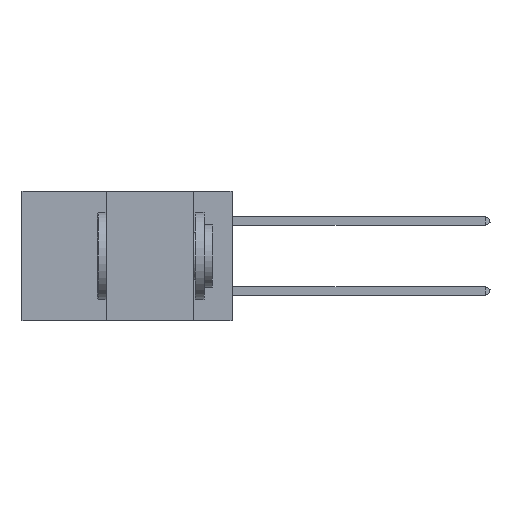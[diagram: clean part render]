
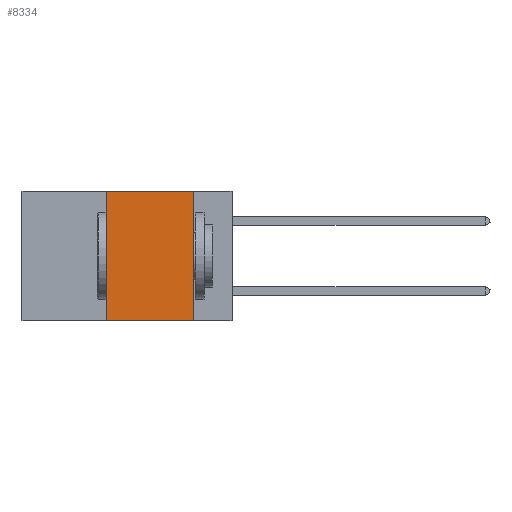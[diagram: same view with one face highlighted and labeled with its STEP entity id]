
A CAD part, left-side view. The second image highlights one B-rep face of the part: STEP entity #8334.
In plain terms, the highlighted planar face has unit normal (-1, 0, 0).
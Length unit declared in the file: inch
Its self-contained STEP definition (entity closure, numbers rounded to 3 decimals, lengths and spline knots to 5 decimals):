
#195 = FACE_OUTER_BOUND ( 'NONE', #5992, .T. ) ;
#325 = VERTEX_POINT ( 'NONE', #12992 ) ;
#503 = DIRECTION ( 'NONE',  ( 0., 0., 1. ) ) ;
#2256 = CARTESIAN_POINT ( 'NONE',  ( 0., 0.36, -0.37 ) ) ;
#2425 = LINE ( 'NONE', #9385, #19684 ) ;
#2683 = CARTESIAN_POINT ( 'NONE',  ( 0., 0.36, 0. ) ) ;
#3695 = EDGE_CURVE ( 'NONE', #325, #13706, #17920, .T. ) ;
#3822 = VERTEX_POINT ( 'NONE', #2256 ) ;
#4269 = EDGE_CURVE ( 'NONE', #20481, #325, #2425, .T. ) ;
#5013 = DIRECTION ( 'NONE',  ( 0., 0., -1. ) ) ;
#5042 = CARTESIAN_POINT ( 'NONE',  ( 0., 0.11, 0. ) ) ;
#5537 = CARTESIAN_POINT ( 'NONE',  ( 0., 0.6, -0.37 ) ) ;
#5992 = EDGE_LOOP ( 'NONE', ( #6625, #15496, #19819, #12196 ) ) ;
#6625 = ORIENTED_EDGE ( 'NONE', *, *, #3695, .F. ) ;
#8334 = ADVANCED_FACE ( 'NONE', ( #195 ), #19979, .F. ) ;
#8519 = DIRECTION ( 'NONE',  ( 0., -1., 0. ) ) ;
#8827 = AXIS2_PLACEMENT_3D ( 'NONE', #16624, #10181, #21620 ) ;
#9231 = VECTOR ( 'NONE', #13923, 39.37008 ) ;
#9385 = CARTESIAN_POINT ( 'NONE',  ( 0., 0.6, 0. ) ) ;
#10110 = CARTESIAN_POINT ( 'NONE',  ( 0., 0.36, 0. ) ) ;
#10181 = DIRECTION ( 'NONE',  ( 1., 0., 0. ) ) ;
#12196 = ORIENTED_EDGE ( 'NONE', *, *, #14826, .T. ) ;
#12992 = CARTESIAN_POINT ( 'NONE',  ( 0., 0.11, 0. ) ) ;
#13103 = VECTOR ( 'NONE', #5013, 39.37008 ) ;
#13273 = VECTOR ( 'NONE', #503, 39.37008 ) ;
#13706 = VERTEX_POINT ( 'NONE', #15265 ) ;
#13923 = DIRECTION ( 'NONE',  ( 0., -1., 0. ) ) ;
#14173 = LINE ( 'NONE', #5537, #9231 ) ;
#14826 = EDGE_CURVE ( 'NONE', #3822, #13706, #14173, .T. ) ;
#15265 = CARTESIAN_POINT ( 'NONE',  ( 0., 0.11, -0.37 ) ) ;
#15496 = ORIENTED_EDGE ( 'NONE', *, *, #4269, .F. ) ;
#16624 = CARTESIAN_POINT ( 'NONE',  ( 0., 0.6, 0. ) ) ;
#17586 = LINE ( 'NONE', #2683, #13273 ) ;
#17609 = EDGE_CURVE ( 'NONE', #3822, #20481, #17586, .T. ) ;
#17920 = LINE ( 'NONE', #5042, #13103 ) ;
#19684 = VECTOR ( 'NONE', #8519, 39.37008 ) ;
#19819 = ORIENTED_EDGE ( 'NONE', *, *, #17609, .F. ) ;
#19979 = PLANE ( 'NONE',  #8827 ) ;
#20481 = VERTEX_POINT ( 'NONE', #10110 ) ;
#21620 = DIRECTION ( 'NONE',  ( 0., 0., -1. ) ) ;
